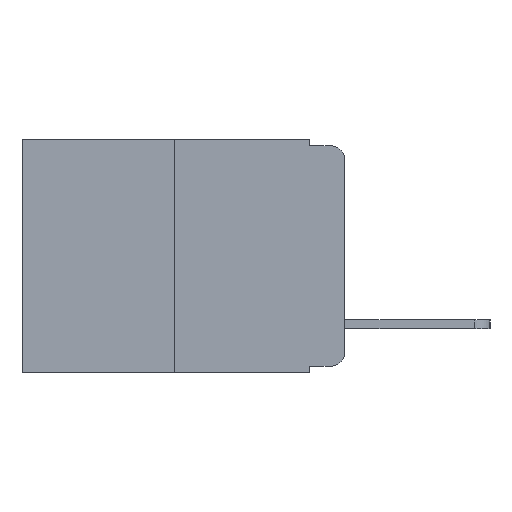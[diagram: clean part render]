
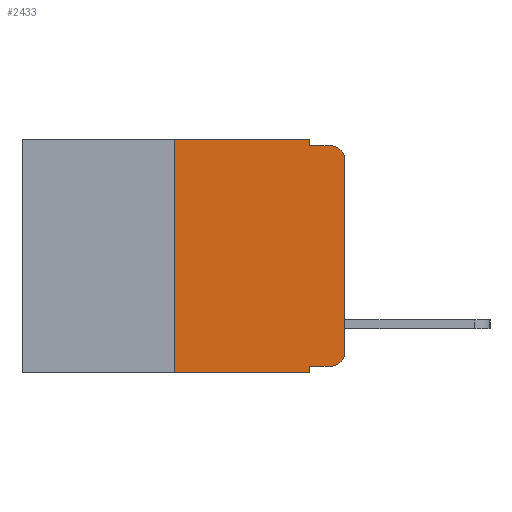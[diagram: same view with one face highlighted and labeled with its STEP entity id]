
A CAD part, left-side view. The second image highlights one B-rep face of the part: STEP entity #2433.
In plain terms, the highlighted planar face has unit normal (-1, 0, 0).
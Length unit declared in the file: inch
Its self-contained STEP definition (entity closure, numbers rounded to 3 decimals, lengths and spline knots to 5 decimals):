
#183 = FACE_OUTER_BOUND ( 'NONE', #6888, .T. ) ;
#196 = ORIENTED_EDGE ( 'NONE', *, *, #3557, .T. ) ;
#288 = DIRECTION ( 'NONE',  ( -1., 0., 0. ) ) ;
#579 = PLANE ( 'NONE',  #4549 ) ;
#760 = AXIS2_PLACEMENT_3D ( 'NONE', #12036, #288, #8810 ) ;
#1120 = VECTOR ( 'NONE', #5069, 39.37008 ) ;
#1313 = VERTEX_POINT ( 'NONE', #3022 ) ;
#1327 = VECTOR ( 'NONE', #4486, 39.37008 ) ;
#1354 = CARTESIAN_POINT ( 'NONE',  ( 0., 0., 0. ) ) ;
#1597 = ORIENTED_EDGE ( 'NONE', *, *, #6987, .T. ) ;
#1859 = CIRCLE ( 'NONE', #3097, 0.02 ) ;
#1996 = CARTESIAN_POINT ( 'NONE',  ( 0., 0.051, 0. ) ) ;
#2244 = CARTESIAN_POINT ( 'NONE',  ( 0., 0., -0.313 ) ) ;
#2433 = ADVANCED_FACE ( 'NONE', ( #183 ), #579, .F. ) ;
#2601 = VECTOR ( 'NONE', #6010, 39.37008 ) ;
#2627 = ORIENTED_EDGE ( 'NONE', *, *, #5445, .T. ) ;
#2810 = VECTOR ( 'NONE', #3858, 39.37008 ) ;
#2820 = CARTESIAN_POINT ( 'NONE',  ( 0., 0.25, 0. ) ) ;
#2888 = EDGE_CURVE ( 'NONE', #3621, #7601, #4591, .T. ) ;
#3022 = CARTESIAN_POINT ( 'NONE',  ( 0., 0.051, -0.333 ) ) ;
#3067 = CARTESIAN_POINT ( 'NONE',  ( 0., 0., -0.03 ) ) ;
#3097 = AXIS2_PLACEMENT_3D ( 'NONE', #3117, #3128, #10090 ) ;
#3110 = CARTESIAN_POINT ( 'NONE',  ( 0., 0.051, 0. ) ) ;
#3117 = CARTESIAN_POINT ( 'NONE',  ( 0., 0.02, -0.03 ) ) ;
#3128 = DIRECTION ( 'NONE',  ( -1., 0., 0. ) ) ;
#3465 = DIRECTION ( 'NONE',  ( 0., 0., -1. ) ) ;
#3557 = EDGE_CURVE ( 'NONE', #6041, #7601, #1859, .T. ) ;
#3572 = ORIENTED_EDGE ( 'NONE', *, *, #5459, .T. ) ;
#3579 = VECTOR ( 'NONE', #8678, 39.37008 ) ;
#3621 = VERTEX_POINT ( 'NONE', #4264 ) ;
#3858 = DIRECTION ( 'NONE',  ( 0., 0., 1. ) ) ;
#3889 = ORIENTED_EDGE ( 'NONE', *, *, #8257, .T. ) ;
#3892 = LINE ( 'NONE', #1996, #3579 ) ;
#3939 = LINE ( 'NONE', #8262, #1327 ) ;
#4161 = CARTESIAN_POINT ( 'NONE',  ( 0., 0.25, -0.343 ) ) ;
#4264 = CARTESIAN_POINT ( 'NONE',  ( 0., 0.051, -0.01 ) ) ;
#4486 = DIRECTION ( 'NONE',  ( 0., -1., 0. ) ) ;
#4549 = AXIS2_PLACEMENT_3D ( 'NONE', #11020, #10822, #10667 ) ;
#4591 = LINE ( 'NONE', #10101, #2601 ) ;
#4736 = VERTEX_POINT ( 'NONE', #3110 ) ;
#5069 = DIRECTION ( 'NONE',  ( 0., -1., 0. ) ) ;
#5206 = VERTEX_POINT ( 'NONE', #2244 ) ;
#5310 = CARTESIAN_POINT ( 'NONE',  ( 0., 0.02, -0.333 ) ) ;
#5352 = LINE ( 'NONE', #2820, #2810 ) ;
#5353 = CARTESIAN_POINT ( 'NONE',  ( 0., 0.051, 0. ) ) ;
#5430 = CARTESIAN_POINT ( 'NONE',  ( 0., 0.02, -0.01 ) ) ;
#5445 = EDGE_CURVE ( 'NONE', #5206, #6041, #11175, .T. ) ;
#5459 = EDGE_CURVE ( 'NONE', #10210, #9125, #8545, .T. ) ;
#5478 = ORIENTED_EDGE ( 'NONE', *, *, #2888, .F. ) ;
#5778 = ORIENTED_EDGE ( 'NONE', *, *, #10185, .F. ) ;
#5991 = VECTOR ( 'NONE', #11614, 39.37008 ) ;
#6010 = DIRECTION ( 'NONE',  ( 0., -1., 0. ) ) ;
#6041 = VERTEX_POINT ( 'NONE', #3067 ) ;
#6076 = ORIENTED_EDGE ( 'NONE', *, *, #10085, .F. ) ;
#6531 = CARTESIAN_POINT ( 'NONE',  ( 0., 0.051, -0.343 ) ) ;
#6888 = EDGE_LOOP ( 'NONE', ( #2627, #196, #5478, #8024, #5778, #10720, #3572, #6076, #3889, #1597 ) ) ;
#6987 = EDGE_CURVE ( 'NONE', #11783, #5206, #11675, .T. ) ;
#7302 = VECTOR ( 'NONE', #3465, 39.37008 ) ;
#7601 = VERTEX_POINT ( 'NONE', #5430 ) ;
#8024 = ORIENTED_EDGE ( 'NONE', *, *, #11813, .F. ) ;
#8257 = EDGE_CURVE ( 'NONE', #1313, #11783, #3939, .T. ) ;
#8262 = CARTESIAN_POINT ( 'NONE',  ( 0., 0.051, -0.333 ) ) ;
#8511 = LINE ( 'NONE', #10628, #1120 ) ;
#8545 = LINE ( 'NONE', #11330, #8831 ) ;
#8678 = DIRECTION ( 'NONE',  ( 0., 0., -1. ) ) ;
#8810 = DIRECTION ( 'NONE',  ( 0., 0., -1. ) ) ;
#8831 = VECTOR ( 'NONE', #11401, 39.37008 ) ;
#9125 = VERTEX_POINT ( 'NONE', #6531 ) ;
#9228 = VERTEX_POINT ( 'NONE', #12117 ) ;
#9481 = LINE ( 'NONE', #5353, #7302 ) ;
#10085 = EDGE_CURVE ( 'NONE', #1313, #9125, #3892, .T. ) ;
#10090 = DIRECTION ( 'NONE',  ( 0., 0., -1. ) ) ;
#10101 = CARTESIAN_POINT ( 'NONE',  ( 0., 0.051, -0.01 ) ) ;
#10185 = EDGE_CURVE ( 'NONE', #9228, #4736, #8511, .T. ) ;
#10210 = VERTEX_POINT ( 'NONE', #4161 ) ;
#10628 = CARTESIAN_POINT ( 'NONE',  ( 0., 0.473, 0. ) ) ;
#10667 = DIRECTION ( 'NONE',  ( 0., 0., -1. ) ) ;
#10671 = EDGE_CURVE ( 'NONE', #10210, #9228, #5352, .T. ) ;
#10720 = ORIENTED_EDGE ( 'NONE', *, *, #10671, .F. ) ;
#10822 = DIRECTION ( 'NONE',  ( 1., 0., 0. ) ) ;
#11020 = CARTESIAN_POINT ( 'NONE',  ( 0., 0.473, 0. ) ) ;
#11175 = LINE ( 'NONE', #1354, #5991 ) ;
#11330 = CARTESIAN_POINT ( 'NONE',  ( 0., 0.473, -0.343 ) ) ;
#11401 = DIRECTION ( 'NONE',  ( 0., -1., 0. ) ) ;
#11614 = DIRECTION ( 'NONE',  ( 0., 0., 1. ) ) ;
#11675 = CIRCLE ( 'NONE', #760, 0.02 ) ;
#11783 = VERTEX_POINT ( 'NONE', #5310 ) ;
#11813 = EDGE_CURVE ( 'NONE', #4736, #3621, #9481, .T. ) ;
#12036 = CARTESIAN_POINT ( 'NONE',  ( 0., 0.02, -0.313 ) ) ;
#12117 = CARTESIAN_POINT ( 'NONE',  ( 0., 0.25, 0. ) ) ;
